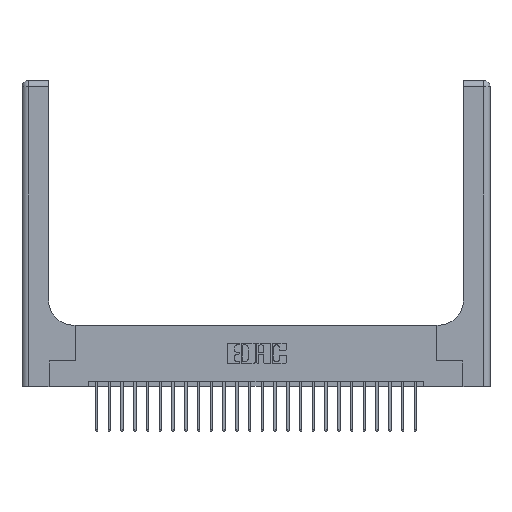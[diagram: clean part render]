
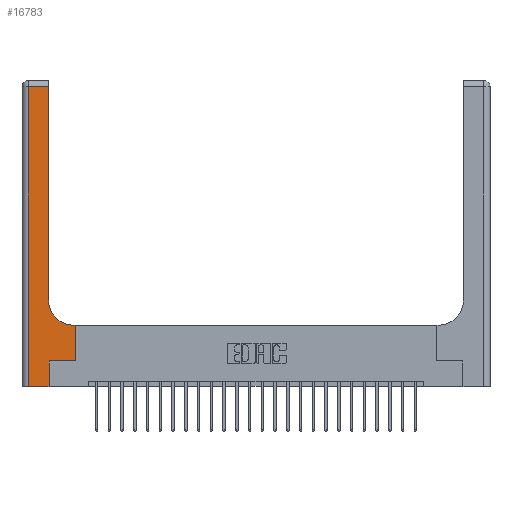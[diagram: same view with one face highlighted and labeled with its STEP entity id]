
A CAD part, top view. The second image highlights one B-rep face of the part: STEP entity #16783.
In plain terms, the highlighted planar face has unit normal (0, 0, 1).
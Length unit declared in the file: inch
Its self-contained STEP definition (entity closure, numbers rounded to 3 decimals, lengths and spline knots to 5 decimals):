
#39 = CARTESIAN_POINT ( 'NONE',  ( 0.528, 0.25, 0.37 ) ) ;
#274 = DIRECTION ( 'NONE',  ( -1., 0., 0. ) ) ;
#479 = DIRECTION ( 'NONE',  ( -1., 0., 0. ) ) ;
#597 = EDGE_CURVE ( 'NONE', #1177, #4831, #19541, .T. ) ;
#651 = CARTESIAN_POINT ( 'NONE',  ( 0.26, 0.6, 0.37 ) ) ;
#664 = EDGE_CURVE ( 'NONE', #4831, #14722, #14510, .T. ) ;
#1165 = VERTEX_POINT ( 'NONE', #7194 ) ;
#1177 = VERTEX_POINT ( 'NONE', #2399 ) ;
#2019 = EDGE_LOOP ( 'NONE', ( #5415, #9671, #11438, #16116, #21729, #5338, #20240, #19324, #18655 ) ) ;
#2399 = CARTESIAN_POINT ( 'NONE',  ( 0.26, 2.94, 0.37 ) ) ;
#2829 = DIRECTION ( 'NONE',  ( 0., 1., 0. ) ) ;
#3358 = FACE_OUTER_BOUND ( 'NONE', #2019, .T. ) ;
#3946 = PLANE ( 'NONE',  #6972 ) ;
#4043 = VECTOR ( 'NONE', #17724, 39.37008 ) ;
#4831 = VERTEX_POINT ( 'NONE', #7714 ) ;
#5324 = DIRECTION ( 'NONE',  ( -1., 0., 0. ) ) ;
#5338 = ORIENTED_EDGE ( 'NONE', *, *, #6516, .T. ) ;
#5415 = ORIENTED_EDGE ( 'NONE', *, *, #20543, .T. ) ;
#5570 = CARTESIAN_POINT ( 'NONE',  ( 0.265, 0.25, 0.37 ) ) ;
#5886 = DIRECTION ( 'NONE',  ( 0., 0., -1. ) ) ;
#6225 = VECTOR ( 'NONE', #22609, 39.37008 ) ;
#6348 = VECTOR ( 'NONE', #5324, 39.37008 ) ;
#6516 = EDGE_CURVE ( 'NONE', #22504, #19880, #9426, .T. ) ;
#6690 = CARTESIAN_POINT ( 'NONE',  ( 0., 0., 0.37 ) ) ;
#6972 = AXIS2_PLACEMENT_3D ( 'NONE', #9867, #5886, #274 ) ;
#7181 = EDGE_CURVE ( 'NONE', #22029, #22504, #18429, .T. ) ;
#7194 = CARTESIAN_POINT ( 'NONE',  ( 0.528, 0.6, 0.37 ) ) ;
#7714 = CARTESIAN_POINT ( 'NONE',  ( 0.06, 2.94, 0.37 ) ) ;
#8005 = CARTESIAN_POINT ( 'NONE',  ( 0.265, 0., 0.37 ) ) ;
#8035 = CARTESIAN_POINT ( 'NONE',  ( 0.26, 3., 0.37 ) ) ;
#8728 = EDGE_CURVE ( 'NONE', #21193, #18984, #17469, .T. ) ;
#9223 = LINE ( 'NONE', #6690, #13597 ) ;
#9393 = EDGE_CURVE ( 'NONE', #1165, #21193, #20759, .T. ) ;
#9426 = LINE ( 'NONE', #5570, #6225 ) ;
#9671 = ORIENTED_EDGE ( 'NONE', *, *, #597, .T. ) ;
#9867 = CARTESIAN_POINT ( 'NONE',  ( 0., 3., 0.37 ) ) ;
#10495 = VECTOR ( 'NONE', #2829, 39.37008 ) ;
#10877 = CARTESIAN_POINT ( 'NONE',  ( 0.06, 0., 0.37 ) ) ;
#11106 = DIRECTION ( 'NONE',  ( 0., -1., 0. ) ) ;
#11438 = ORIENTED_EDGE ( 'NONE', *, *, #664, .T. ) ;
#11817 = DIRECTION ( 'NONE',  ( 1., 0., 0. ) ) ;
#13062 = VECTOR ( 'NONE', #479, 39.37008 ) ;
#13462 = LINE ( 'NONE', #8035, #21177 ) ;
#13597 = VECTOR ( 'NONE', #17904, 39.37008 ) ;
#13760 = EDGE_CURVE ( 'NONE', #19880, #1165, #24072, .T. ) ;
#14231 = VECTOR ( 'NONE', #11106, 39.37008 ) ;
#14510 = LINE ( 'NONE', #24081, #14231 ) ;
#14722 = VERTEX_POINT ( 'NONE', #10877 ) ;
#14736 = CARTESIAN_POINT ( 'NONE',  ( 0.26, 0.85, 0.37 ) ) ;
#15548 = DIRECTION ( 'NONE',  ( 0., 1., 0. ) ) ;
#15965 = AXIS2_PLACEMENT_3D ( 'NONE', #21262, #19059, #11817 ) ;
#16116 = ORIENTED_EDGE ( 'NONE', *, *, #16980, .T. ) ;
#16146 = CARTESIAN_POINT ( 'NONE',  ( 0.51, 0.6, 0.37 ) ) ;
#16594 = CARTESIAN_POINT ( 'NONE',  ( 0., 2.94, 0.37 ) ) ;
#16783 = ADVANCED_FACE ( 'NONE', ( #3358 ), #3946, .F. ) ;
#16980 = EDGE_CURVE ( 'NONE', #14722, #22029, #9223, .T. ) ;
#17469 = CIRCLE ( 'NONE', #15965, 0.25 ) ;
#17600 = CARTESIAN_POINT ( 'NONE',  ( 0.265, 0., 0.37 ) ) ;
#17724 = DIRECTION ( 'NONE',  ( 0., 1., 0. ) ) ;
#17904 = DIRECTION ( 'NONE',  ( 1., 0., 0. ) ) ;
#18429 = LINE ( 'NONE', #17600, #10495 ) ;
#18655 = ORIENTED_EDGE ( 'NONE', *, *, #8728, .T. ) ;
#18984 = VERTEX_POINT ( 'NONE', #14736 ) ;
#19059 = DIRECTION ( 'NONE',  ( 0., 0., -1. ) ) ;
#19324 = ORIENTED_EDGE ( 'NONE', *, *, #9393, .T. ) ;
#19541 = LINE ( 'NONE', #16594, #6348 ) ;
#19880 = VERTEX_POINT ( 'NONE', #39 ) ;
#20240 = ORIENTED_EDGE ( 'NONE', *, *, #13760, .T. ) ;
#20543 = EDGE_CURVE ( 'NONE', #18984, #1177, #13462, .T. ) ;
#20759 = LINE ( 'NONE', #651, #13062 ) ;
#21177 = VECTOR ( 'NONE', #15548, 39.37008 ) ;
#21193 = VERTEX_POINT ( 'NONE', #16146 ) ;
#21262 = CARTESIAN_POINT ( 'NONE',  ( 0.51, 0.85, 0.37 ) ) ;
#21434 = CARTESIAN_POINT ( 'NONE',  ( 0.528, 0.25, 0.37 ) ) ;
#21680 = CARTESIAN_POINT ( 'NONE',  ( 0.265, 0.25, 0.37 ) ) ;
#21729 = ORIENTED_EDGE ( 'NONE', *, *, #7181, .T. ) ;
#22029 = VERTEX_POINT ( 'NONE', #8005 ) ;
#22504 = VERTEX_POINT ( 'NONE', #21680 ) ;
#22609 = DIRECTION ( 'NONE',  ( 1., 0., 0. ) ) ;
#24072 = LINE ( 'NONE', #21434, #4043 ) ;
#24081 = CARTESIAN_POINT ( 'NONE',  ( 0.06, 3., 0.37 ) ) ;
